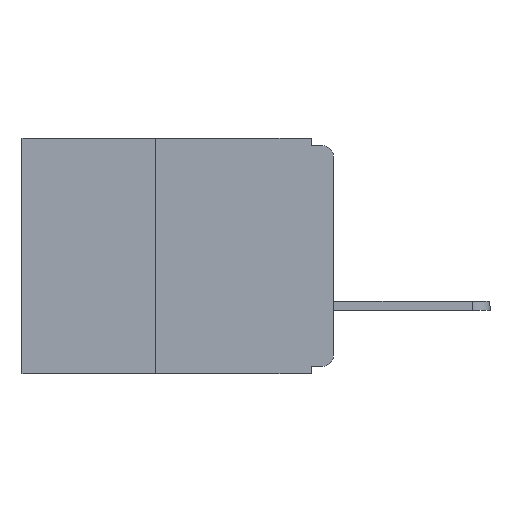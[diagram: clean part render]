
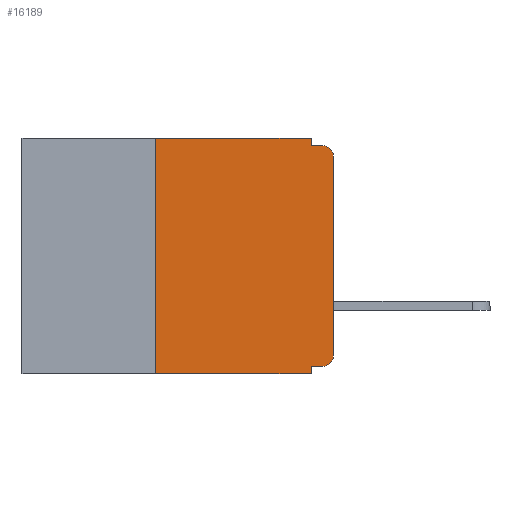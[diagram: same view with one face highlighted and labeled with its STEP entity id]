
A CAD part, left-side view. The second image highlights one B-rep face of the part: STEP entity #16189.
In plain terms, the highlighted planar face has unit normal (-1, 0, 0).
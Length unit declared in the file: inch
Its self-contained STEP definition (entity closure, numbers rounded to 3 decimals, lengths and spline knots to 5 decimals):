
#260 = CIRCLE ( 'NONE', #3779, 0.015 ) ;
#329 = VECTOR ( 'NONE', #13289, 39.37008 ) ;
#1475 = VERTEX_POINT ( 'NONE', #20184 ) ;
#1665 = CARTESIAN_POINT ( 'NONE',  ( 0., 0., -0.305 ) ) ;
#2519 = LINE ( 'NONE', #4120, #12936 ) ;
#2928 = CARTESIAN_POINT ( 'NONE',  ( 0., 0.015, -0.025 ) ) ;
#3266 = CARTESIAN_POINT ( 'NONE',  ( 0., 0., 0. ) ) ;
#3779 = AXIS2_PLACEMENT_3D ( 'NONE', #2928, #18424, #5173 ) ;
#4106 = EDGE_CURVE ( 'NONE', #9404, #5205, #23263, .T. ) ;
#4120 = CARTESIAN_POINT ( 'NONE',  ( 0., 0.031, -0.33 ) ) ;
#5173 = DIRECTION ( 'NONE',  ( 0., 0., -1. ) ) ;
#5186 = CARTESIAN_POINT ( 'NONE',  ( 0., 0.25, -0.33 ) ) ;
#5205 = VERTEX_POINT ( 'NONE', #17000 ) ;
#5378 = VERTEX_POINT ( 'NONE', #26447 ) ;
#5433 = VERTEX_POINT ( 'NONE', #17675 ) ;
#5751 = EDGE_CURVE ( 'NONE', #18470, #14957, #25239, .T. ) ;
#6458 = ORIENTED_EDGE ( 'NONE', *, *, #24623, .T. ) ;
#6463 = CARTESIAN_POINT ( 'NONE',  ( 0., 0.031, -0.32 ) ) ;
#7307 = CARTESIAN_POINT ( 'NONE',  ( 0., 0.437, 0. ) ) ;
#8553 = CARTESIAN_POINT ( 'NONE',  ( 0., 0.015, -0.305 ) ) ;
#8814 = VECTOR ( 'NONE', #24845, 39.37008 ) ;
#9061 = DIRECTION ( 'NONE',  ( 0., -1., 0. ) ) ;
#9170 = DIRECTION ( 'NONE',  ( 0., 0., -1. ) ) ;
#9404 = VERTEX_POINT ( 'NONE', #28044 ) ;
#9414 = EDGE_CURVE ( 'NONE', #5205, #5433, #13908, .T. ) ;
#9738 = DIRECTION ( 'NONE',  ( 0., 0., 1. ) ) ;
#10412 = DIRECTION ( 'NONE',  ( 0., -1., 0. ) ) ;
#10743 = DIRECTION ( 'NONE',  ( 0., 0., -1. ) ) ;
#10801 = ORIENTED_EDGE ( 'NONE', *, *, #4106, .F. ) ;
#10916 = VERTEX_POINT ( 'NONE', #26996 ) ;
#11462 = EDGE_CURVE ( 'NONE', #14957, #5433, #260, .T. ) ;
#11559 = EDGE_CURVE ( 'NONE', #19762, #10916, #20390, .T. ) ;
#12118 = DIRECTION ( 'NONE',  ( 0., 0., 1. ) ) ;
#12163 = DIRECTION ( 'NONE',  ( 0., -1., 0. ) ) ;
#12213 = ORIENTED_EDGE ( 'NONE', *, *, #5751, .T. ) ;
#12769 = AXIS2_PLACEMENT_3D ( 'NONE', #7307, #22452, #9170 ) ;
#12936 = VECTOR ( 'NONE', #21859, 39.37008 ) ;
#13289 = DIRECTION ( 'NONE',  ( 0., 0., -1. ) ) ;
#13405 = VECTOR ( 'NONE', #9738, 39.37008 ) ;
#13629 = ORIENTED_EDGE ( 'NONE', *, *, #24194, .T. ) ;
#13908 = LINE ( 'NONE', #21506, #24347 ) ;
#14326 = CARTESIAN_POINT ( 'NONE',  ( 0., 0.25, -0.33 ) ) ;
#14725 = CARTESIAN_POINT ( 'NONE',  ( 0., 0.031, 0. ) ) ;
#14957 = VERTEX_POINT ( 'NONE', #25022 ) ;
#15194 = ORIENTED_EDGE ( 'NONE', *, *, #16654, .F. ) ;
#15415 = ORIENTED_EDGE ( 'NONE', *, *, #9414, .F. ) ;
#16074 = PLANE ( 'NONE',  #12769 ) ;
#16189 = ADVANCED_FACE ( 'NONE', ( #20980 ), #16074, .F. ) ;
#16654 = EDGE_CURVE ( 'NONE', #27170, #5378, #2519, .T. ) ;
#17000 = CARTESIAN_POINT ( 'NONE',  ( 0., 0.031, -0.01 ) ) ;
#17620 = ORIENTED_EDGE ( 'NONE', *, *, #11559, .F. ) ;
#17675 = CARTESIAN_POINT ( 'NONE',  ( 0., 0.015, -0.01 ) ) ;
#17844 = CARTESIAN_POINT ( 'NONE',  ( 0., 0.437, 0. ) ) ;
#18066 = EDGE_CURVE ( 'NONE', #10916, #9404, #22269, .T. ) ;
#18165 = ORIENTED_EDGE ( 'NONE', *, *, #26087, .F. ) ;
#18424 = DIRECTION ( 'NONE',  ( -1., 0., 0. ) ) ;
#18470 = VERTEX_POINT ( 'NONE', #1665 ) ;
#18761 = CARTESIAN_POINT ( 'NONE',  ( 0., 0.437, -0.33 ) ) ;
#19762 = VERTEX_POINT ( 'NONE', #5186 ) ;
#20184 = CARTESIAN_POINT ( 'NONE',  ( 0., 0.015, -0.32 ) ) ;
#20390 = LINE ( 'NONE', #14326, #25609 ) ;
#20599 = LINE ( 'NONE', #22590, #8814 ) ;
#20980 = FACE_OUTER_BOUND ( 'NONE', #27536, .T. ) ;
#21506 = CARTESIAN_POINT ( 'NONE',  ( 0., 0., -0.01 ) ) ;
#21859 = DIRECTION ( 'NONE',  ( 0., 0., -1. ) ) ;
#22194 = CIRCLE ( 'NONE', #27423, 0.015 ) ;
#22269 = LINE ( 'NONE', #17844, #22972 ) ;
#22452 = DIRECTION ( 'NONE',  ( 1., 0., 0. ) ) ;
#22590 = CARTESIAN_POINT ( 'NONE',  ( 0., 0., -0.32 ) ) ;
#22871 = LINE ( 'NONE', #18761, #26654 ) ;
#22972 = VECTOR ( 'NONE', #9061, 39.37008 ) ;
#23263 = LINE ( 'NONE', #14725, #329 ) ;
#23530 = ORIENTED_EDGE ( 'NONE', *, *, #11462, .T. ) ;
#24046 = DIRECTION ( 'NONE',  ( -1., 0., 0. ) ) ;
#24194 = EDGE_CURVE ( 'NONE', #1475, #18470, #22194, .T. ) ;
#24347 = VECTOR ( 'NONE', #10412, 39.37008 ) ;
#24623 = EDGE_CURVE ( 'NONE', #19762, #5378, #22871, .T. ) ;
#24845 = DIRECTION ( 'NONE',  ( 0., 1., 0. ) ) ;
#25022 = CARTESIAN_POINT ( 'NONE',  ( 0., 0., -0.025 ) ) ;
#25239 = LINE ( 'NONE', #3266, #13405 ) ;
#25609 = VECTOR ( 'NONE', #12118, 39.37008 ) ;
#25823 = ORIENTED_EDGE ( 'NONE', *, *, #18066, .F. ) ;
#26087 = EDGE_CURVE ( 'NONE', #1475, #27170, #20599, .T. ) ;
#26447 = CARTESIAN_POINT ( 'NONE',  ( 0., 0.031, -0.33 ) ) ;
#26654 = VECTOR ( 'NONE', #12163, 39.37008 ) ;
#26996 = CARTESIAN_POINT ( 'NONE',  ( 0., 0.25, 0. ) ) ;
#27170 = VERTEX_POINT ( 'NONE', #6463 ) ;
#27423 = AXIS2_PLACEMENT_3D ( 'NONE', #8553, #24046, #10743 ) ;
#27536 = EDGE_LOOP ( 'NONE', ( #12213, #23530, #15415, #10801, #25823, #17620, #6458, #15194, #18165, #13629 ) ) ;
#28044 = CARTESIAN_POINT ( 'NONE',  ( 0., 0.031, 0. ) ) ;
